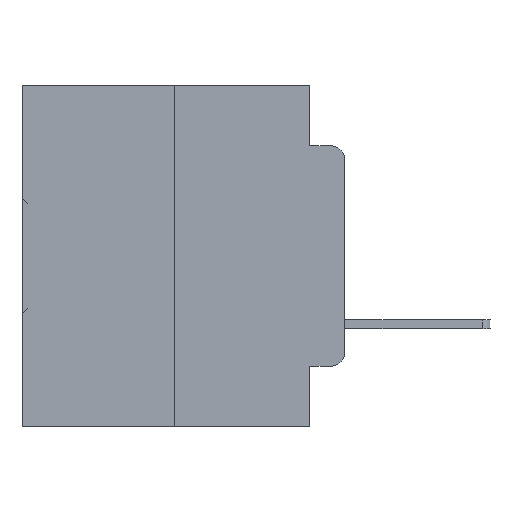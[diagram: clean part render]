
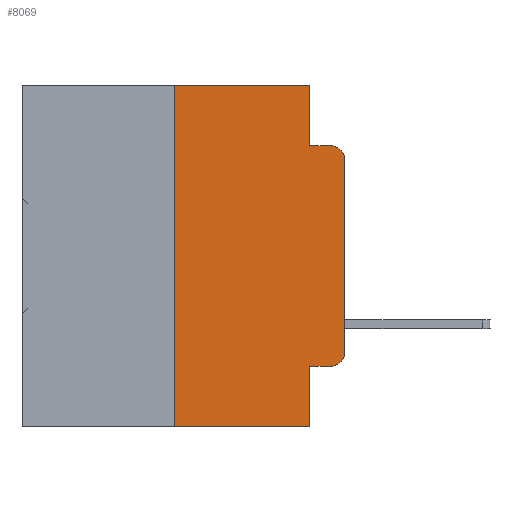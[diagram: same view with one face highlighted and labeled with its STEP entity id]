
A CAD part, left-side view. The second image highlights one B-rep face of the part: STEP entity #8069.
In plain terms, the highlighted planar face has unit normal (-1, 0, 0).
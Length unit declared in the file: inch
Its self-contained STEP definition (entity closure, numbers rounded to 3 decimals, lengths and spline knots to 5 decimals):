
#69 = LINE ( 'NONE', #13934, #27708 ) ;
#1748 = DIRECTION ( 'NONE',  ( 0., -1., 0. ) ) ;
#1757 = PLANE ( 'NONE',  #13613 ) ;
#4222 = VECTOR ( 'NONE', #1748, 39.37008 ) ;
#5258 = ORIENTED_EDGE ( 'NONE', *, *, #8860, .F. ) ;
#5271 = EDGE_CURVE ( 'NONE', #21564, #24706, #33229, .T. ) ;
#5556 = CARTESIAN_POINT ( 'NONE',  ( 0., 0.02, -0.4115 ) ) ;
#5584 = AXIS2_PLACEMENT_3D ( 'NONE', #12719, #30508, #15322 ) ;
#5703 = CARTESIAN_POINT ( 'NONE',  ( 0., 0.02, -0.1085 ) ) ;
#5908 = CARTESIAN_POINT ( 'NONE',  ( 0., 0.051, 0. ) ) ;
#6702 = LINE ( 'NONE', #5908, #26477 ) ;
#6924 = ORIENTED_EDGE ( 'NONE', *, *, #5271, .F. ) ;
#7114 = CARTESIAN_POINT ( 'NONE',  ( 0., 0.473, 0. ) ) ;
#8069 = ADVANCED_FACE ( 'NONE', ( #9029 ), #1757, .F. ) ;
#8098 = DIRECTION ( 'NONE',  ( 0., 0., 1. ) ) ;
#8401 = DIRECTION ( 'NONE',  ( 0., 0., -1. ) ) ;
#8860 = EDGE_CURVE ( 'NONE', #16972, #15829, #19121, .T. ) ;
#8915 = CARTESIAN_POINT ( 'NONE',  ( 0., 0.02, -0.0885 ) ) ;
#9029 = FACE_OUTER_BOUND ( 'NONE', #32608, .T. ) ;
#9844 = DIRECTION ( 'NONE',  ( 0., 0., -1. ) ) ;
#10317 = VERTEX_POINT ( 'NONE', #33550 ) ;
#10708 = ORIENTED_EDGE ( 'NONE', *, *, #11749, .F. ) ;
#10713 = VERTEX_POINT ( 'NONE', #30066 ) ;
#11104 = CARTESIAN_POINT ( 'NONE',  ( 0., 0.25, 0. ) ) ;
#11322 = LINE ( 'NONE', #32689, #4222 ) ;
#11749 = EDGE_CURVE ( 'NONE', #10317, #23833, #6702, .T. ) ;
#12486 = DIRECTION ( 'NONE',  ( 0., 0., -1. ) ) ;
#12719 = CARTESIAN_POINT ( 'NONE',  ( 0., 0.02, -0.3915 ) ) ;
#13613 = AXIS2_PLACEMENT_3D ( 'NONE', #7114, #25178, #9844 ) ;
#13900 = VECTOR ( 'NONE', #15478, 39.37008 ) ;
#13934 = CARTESIAN_POINT ( 'NONE',  ( 0., 0.473, 0. ) ) ;
#14356 = ORIENTED_EDGE ( 'NONE', *, *, #24804, .T. ) ;
#15322 = DIRECTION ( 'NONE',  ( 0., 0., -1. ) ) ;
#15323 = VECTOR ( 'NONE', #8098, 39.37008 ) ;
#15440 = VERTEX_POINT ( 'NONE', #8915 ) ;
#15478 = DIRECTION ( 'NONE',  ( 0., 0., 1. ) ) ;
#15829 = VERTEX_POINT ( 'NONE', #11104 ) ;
#15902 = CARTESIAN_POINT ( 'NONE',  ( 0., 0., 0. ) ) ;
#16118 = EDGE_CURVE ( 'NONE', #16972, #24706, #11322, .T. ) ;
#16848 = CIRCLE ( 'NONE', #5584, 0.02 ) ;
#16972 = VERTEX_POINT ( 'NONE', #26109 ) ;
#17660 = VERTEX_POINT ( 'NONE', #28815 ) ;
#17750 = DIRECTION ( 'NONE',  ( 0., -1., 0. ) ) ;
#18049 = EDGE_CURVE ( 'NONE', #23833, #15440, #31127, .T. ) ;
#18162 = CARTESIAN_POINT ( 'NONE',  ( 0., 0.051, -0.5 ) ) ;
#19121 = LINE ( 'NONE', #33213, #13900 ) ;
#19189 = ORIENTED_EDGE ( 'NONE', *, *, #16118, .T. ) ;
#19524 = CARTESIAN_POINT ( 'NONE',  ( 0., 0.051, -0.4115 ) ) ;
#20791 = ORIENTED_EDGE ( 'NONE', *, *, #30074, .T. ) ;
#21564 = VERTEX_POINT ( 'NONE', #32679 ) ;
#22088 = LINE ( 'NONE', #15902, #15323 ) ;
#23124 = EDGE_CURVE ( 'NONE', #10713, #15440, #25737, .T. ) ;
#23530 = ORIENTED_EDGE ( 'NONE', *, *, #18049, .F. ) ;
#23833 = VERTEX_POINT ( 'NONE', #29240 ) ;
#23838 = DIRECTION ( 'NONE',  ( -1., 0., 0. ) ) ;
#24119 = VECTOR ( 'NONE', #32087, 39.37008 ) ;
#24706 = VERTEX_POINT ( 'NONE', #18162 ) ;
#24804 = EDGE_CURVE ( 'NONE', #17660, #10713, #22088, .T. ) ;
#24920 = LINE ( 'NONE', #19524, #24119 ) ;
#25178 = DIRECTION ( 'NONE',  ( 1., 0., 0. ) ) ;
#25276 = CARTESIAN_POINT ( 'NONE',  ( 0., 0.051, -0.0885 ) ) ;
#25737 = CIRCLE ( 'NONE', #29464, 0.02 ) ;
#26109 = CARTESIAN_POINT ( 'NONE',  ( 0., 0.25, -0.5 ) ) ;
#26477 = VECTOR ( 'NONE', #31448, 39.37008 ) ;
#26690 = EDGE_CURVE ( 'NONE', #27486, #17660, #16848, .T. ) ;
#27276 = VECTOR ( 'NONE', #12486, 39.37008 ) ;
#27486 = VERTEX_POINT ( 'NONE', #5556 ) ;
#27708 = VECTOR ( 'NONE', #29150, 39.37008 ) ;
#28648 = ORIENTED_EDGE ( 'NONE', *, *, #23124, .T. ) ;
#28815 = CARTESIAN_POINT ( 'NONE',  ( 0., 0., -0.3915 ) ) ;
#29058 = ORIENTED_EDGE ( 'NONE', *, *, #26690, .T. ) ;
#29150 = DIRECTION ( 'NONE',  ( 0., -1., 0. ) ) ;
#29240 = CARTESIAN_POINT ( 'NONE',  ( 0., 0.051, -0.0885 ) ) ;
#29464 = AXIS2_PLACEMENT_3D ( 'NONE', #5703, #23838, #8401 ) ;
#30066 = CARTESIAN_POINT ( 'NONE',  ( 0., 0., -0.1085 ) ) ;
#30074 = EDGE_CURVE ( 'NONE', #21564, #27486, #24920, .T. ) ;
#30274 = CARTESIAN_POINT ( 'NONE',  ( 0., 0.051, 0. ) ) ;
#30508 = DIRECTION ( 'NONE',  ( -1., 0., 0. ) ) ;
#31127 = LINE ( 'NONE', #25276, #31877 ) ;
#31211 = EDGE_CURVE ( 'NONE', #15829, #10317, #69, .T. ) ;
#31448 = DIRECTION ( 'NONE',  ( 0., 0., -1. ) ) ;
#31804 = ORIENTED_EDGE ( 'NONE', *, *, #31211, .F. ) ;
#31877 = VECTOR ( 'NONE', #17750, 39.37008 ) ;
#32087 = DIRECTION ( 'NONE',  ( 0., -1., 0. ) ) ;
#32608 = EDGE_LOOP ( 'NONE', ( #14356, #28648, #23530, #10708, #31804, #5258, #19189, #6924, #20791, #29058 ) ) ;
#32679 = CARTESIAN_POINT ( 'NONE',  ( 0., 0.051, -0.4115 ) ) ;
#32689 = CARTESIAN_POINT ( 'NONE',  ( 0., 0.473, -0.5 ) ) ;
#33213 = CARTESIAN_POINT ( 'NONE',  ( 0., 0.25, 0. ) ) ;
#33229 = LINE ( 'NONE', #30274, #27276 ) ;
#33550 = CARTESIAN_POINT ( 'NONE',  ( 0., 0.051, 0. ) ) ;
